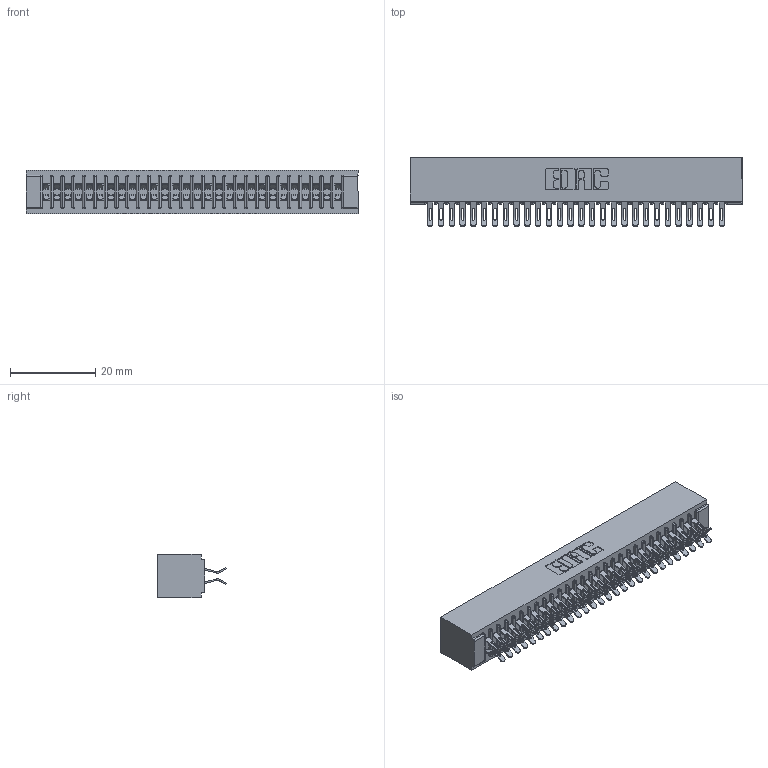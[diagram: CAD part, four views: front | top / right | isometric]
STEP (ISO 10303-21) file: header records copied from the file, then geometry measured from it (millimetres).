
FILE_DESCRIPTION (( 'STEP AP203' ), '1' );
FILE_NAME ('341-056-555-201.STEP', '2018-08-07T15:27:24', ( '' ), ( '' ), 'SwSTEP 2.0', 'SolidWorks 2016', '' );
FILE_SCHEMA (( 'CONFIG_CONTROL_DESIGN' ));
Length unit declared in the file: inch
Products named in the file (3): 341-056-555-201; 341 Part_No Mounting Lugs; 341-292-001_341-292-155
Assembly tree (57 placements, depth 2):
  341-056-555-201
    341 Part_No Mounting Lugs
    341-292-001_341-292-155  x56
Bounding box: 78.11 x 16.31 x 10.16 mm (x, y, z)
Volume: 6062.3 mm3; surface area: 11438.7 mm2
Topology: 57 solids, 57 shells, 4476 faces, 13368 edges, 8702 vertices
Faces by surface type: plane 2416, cylinder 1948, sphere 58, torus 54
Entity records: 35943 total; most frequent: CARTESIAN_POINT 5990, ORIENTED_EDGE 5940, DIRECTION 5812, EDGE_CURVE 2970, LINE 2372, VECTOR 2372, VERTEX_POINT 1882, AXIS2_PLACEMENT_3D 1720
